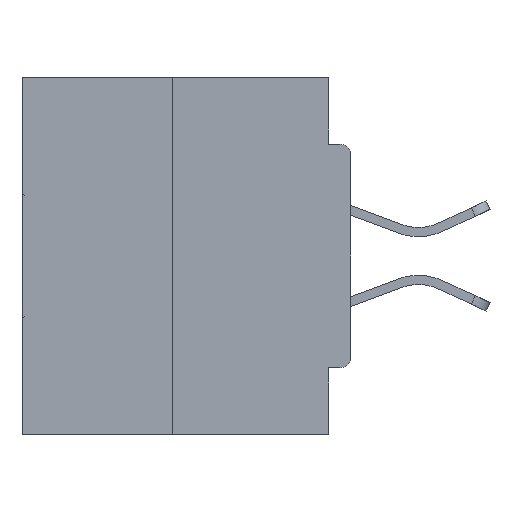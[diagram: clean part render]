
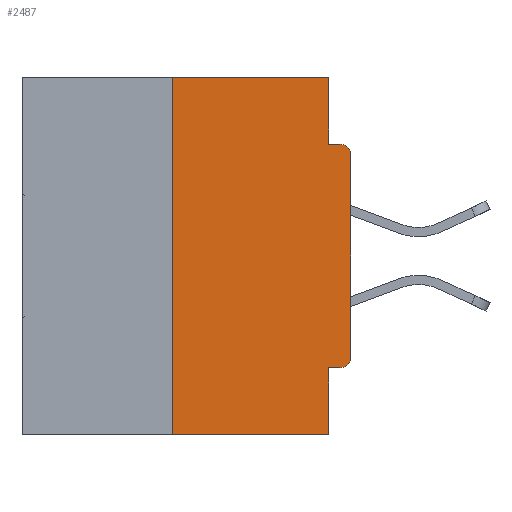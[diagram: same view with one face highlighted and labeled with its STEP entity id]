
A CAD part, left-side view. The second image highlights one B-rep face of the part: STEP entity #2487.
In plain terms, the highlighted planar face has unit normal (-1, 0, 0).
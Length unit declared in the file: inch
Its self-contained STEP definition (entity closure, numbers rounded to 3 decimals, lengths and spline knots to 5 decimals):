
#593 = EDGE_CURVE ( 'NONE', #16955, #24825, #32693, .T. ) ;
#862 = DIRECTION ( 'NONE',  ( 0., 0., -1. ) ) ;
#866 = VERTEX_POINT ( 'NONE', #16472 ) ;
#2258 = VERTEX_POINT ( 'NONE', #23929 ) ;
#2487 = ADVANCED_FACE ( 'NONE', ( #14314 ), #33657, .F. ) ;
#2919 = VERTEX_POINT ( 'NONE', #36304 ) ;
#3290 = DIRECTION ( 'NONE',  ( 0., -1., 0. ) ) ;
#3297 = ORIENTED_EDGE ( 'NONE', *, *, #28475, .T. ) ;
#3715 = DIRECTION ( 'NONE',  ( 0., -1., 0. ) ) ;
#4456 = AXIS2_PLACEMENT_3D ( 'NONE', #19582, #22825, #33081 ) ;
#4496 = VERTEX_POINT ( 'NONE', #23605 ) ;
#4602 = VECTOR ( 'NONE', #3715, 39.37008 ) ;
#6110 = ORIENTED_EDGE ( 'NONE', *, *, #37438, .F. ) ;
#6666 = CARTESIAN_POINT ( 'NONE',  ( 0., 0.031, -0.5 ) ) ;
#6901 = LINE ( 'NONE', #10526, #29715 ) ;
#8327 = CARTESIAN_POINT ( 'NONE',  ( 0., 0., -0.1085 ) ) ;
#8479 = VERTEX_POINT ( 'NONE', #34378 ) ;
#8786 = EDGE_CURVE ( 'NONE', #4496, #866, #41553, .T. ) ;
#9223 = DIRECTION ( 'NONE',  ( -1., 0., 0. ) ) ;
#9800 = CARTESIAN_POINT ( 'NONE',  ( 0., 0.46, 0. ) ) ;
#9842 = VECTOR ( 'NONE', #34578, 39.37008 ) ;
#10526 = CARTESIAN_POINT ( 'NONE',  ( 0., 0.031, -0.5 ) ) ;
#10695 = CARTESIAN_POINT ( 'NONE',  ( 0., 0.46, 0. ) ) ;
#10712 = ORIENTED_EDGE ( 'NONE', *, *, #23148, .T. ) ;
#10717 = VECTOR ( 'NONE', #16283, 39.37008 ) ;
#11093 = CARTESIAN_POINT ( 'NONE',  ( 0., 0.015, -0.0935 ) ) ;
#11880 = DIRECTION ( 'NONE',  ( 0., 0., 1. ) ) ;
#12344 = DIRECTION ( 'NONE',  ( 0., 0., -1. ) ) ;
#12503 = ORIENTED_EDGE ( 'NONE', *, *, #8786, .F. ) ;
#13366 = EDGE_CURVE ( 'NONE', #2919, #18357, #18808, .T. ) ;
#14194 = ORIENTED_EDGE ( 'NONE', *, *, #19080, .F. ) ;
#14314 = FACE_OUTER_BOUND ( 'NONE', #40951, .T. ) ;
#14872 = ORIENTED_EDGE ( 'NONE', *, *, #13366, .F. ) ;
#15290 = CARTESIAN_POINT ( 'NONE',  ( 0., 0., -0.4065 ) ) ;
#15920 = CARTESIAN_POINT ( 'NONE',  ( 0., 0.031, 0. ) ) ;
#16283 = DIRECTION ( 'NONE',  ( 0., -1., 0. ) ) ;
#16472 = CARTESIAN_POINT ( 'NONE',  ( 0., 0.031, -0.4065 ) ) ;
#16632 = CARTESIAN_POINT ( 'NONE',  ( 0., 0.46, -0.5 ) ) ;
#16955 = VERTEX_POINT ( 'NONE', #34234 ) ;
#18129 = CARTESIAN_POINT ( 'NONE',  ( 0., 0.25, 0. ) ) ;
#18263 = ORIENTED_EDGE ( 'NONE', *, *, #21306, .F. ) ;
#18357 = VERTEX_POINT ( 'NONE', #11093 ) ;
#18808 = LINE ( 'NONE', #38768, #33072 ) ;
#19080 = EDGE_CURVE ( 'NONE', #2258, #2919, #20512, .T. ) ;
#19582 = CARTESIAN_POINT ( 'NONE',  ( 0., 0.015, -0.3915 ) ) ;
#20512 = LINE ( 'NONE', #15920, #22024 ) ;
#21306 = EDGE_CURVE ( 'NONE', #27442, #2258, #31982, .T. ) ;
#22024 = VECTOR ( 'NONE', #25714, 39.37008 ) ;
#22435 = VERTEX_POINT ( 'NONE', #6666 ) ;
#22825 = DIRECTION ( 'NONE',  ( -1., 0., 0. ) ) ;
#23148 = EDGE_CURVE ( 'NONE', #24825, #18357, #33415, .T. ) ;
#23605 = CARTESIAN_POINT ( 'NONE',  ( 0., 0.015, -0.4065 ) ) ;
#23929 = CARTESIAN_POINT ( 'NONE',  ( 0., 0.031, 0. ) ) ;
#24825 = VERTEX_POINT ( 'NONE', #8327 ) ;
#25705 = CIRCLE ( 'NONE', #4456, 0.015 ) ;
#25714 = DIRECTION ( 'NONE',  ( 0., 0., -1. ) ) ;
#27442 = VERTEX_POINT ( 'NONE', #27748 ) ;
#27748 = CARTESIAN_POINT ( 'NONE',  ( 0., 0.25, 0. ) ) ;
#28435 = CARTESIAN_POINT ( 'NONE',  ( 0., 0., 0. ) ) ;
#28475 = EDGE_CURVE ( 'NONE', #8479, #22435, #30486, .T. ) ;
#29715 = VECTOR ( 'NONE', #33201, 39.37008 ) ;
#29847 = DIRECTION ( 'NONE',  ( 0., 1., 0. ) ) ;
#30486 = LINE ( 'NONE', #16632, #4602 ) ;
#31982 = LINE ( 'NONE', #9800, #10717 ) ;
#32693 = LINE ( 'NONE', #28435, #38259 ) ;
#32791 = AXIS2_PLACEMENT_3D ( 'NONE', #34875, #9223, #12344 ) ;
#33072 = VECTOR ( 'NONE', #3290, 39.37008 ) ;
#33081 = DIRECTION ( 'NONE',  ( 0., 0., -1. ) ) ;
#33201 = DIRECTION ( 'NONE',  ( 0., 0., -1. ) ) ;
#33415 = CIRCLE ( 'NONE', #32791, 0.015 ) ;
#33514 = DIRECTION ( 'NONE',  ( 1., 0., 0. ) ) ;
#33657 = PLANE ( 'NONE',  #34850 ) ;
#33948 = VECTOR ( 'NONE', #29847, 39.37008 ) ;
#34234 = CARTESIAN_POINT ( 'NONE',  ( 0., 0., -0.3915 ) ) ;
#34378 = CARTESIAN_POINT ( 'NONE',  ( 0., 0.25, -0.5 ) ) ;
#34578 = DIRECTION ( 'NONE',  ( 0., 0., 1. ) ) ;
#34850 = AXIS2_PLACEMENT_3D ( 'NONE', #10695, #33514, #862 ) ;
#34875 = CARTESIAN_POINT ( 'NONE',  ( 0., 0.015, -0.1085 ) ) ;
#35477 = ORIENTED_EDGE ( 'NONE', *, *, #41869, .F. ) ;
#36304 = CARTESIAN_POINT ( 'NONE',  ( 0., 0.031, -0.0935 ) ) ;
#36714 = ORIENTED_EDGE ( 'NONE', *, *, #593, .T. ) ;
#37438 = EDGE_CURVE ( 'NONE', #8479, #27442, #41300, .T. ) ;
#38259 = VECTOR ( 'NONE', #11880, 39.37008 ) ;
#38768 = CARTESIAN_POINT ( 'NONE',  ( 0., 0., -0.0935 ) ) ;
#40951 = EDGE_LOOP ( 'NONE', ( #18263, #6110, #3297, #35477, #12503, #41693, #36714, #10712, #14872, #14194 ) ) ;
#41001 = EDGE_CURVE ( 'NONE', #4496, #16955, #25705, .T. ) ;
#41300 = LINE ( 'NONE', #18129, #9842 ) ;
#41553 = LINE ( 'NONE', #15290, #33948 ) ;
#41693 = ORIENTED_EDGE ( 'NONE', *, *, #41001, .T. ) ;
#41869 = EDGE_CURVE ( 'NONE', #866, #22435, #6901, .T. ) ;
